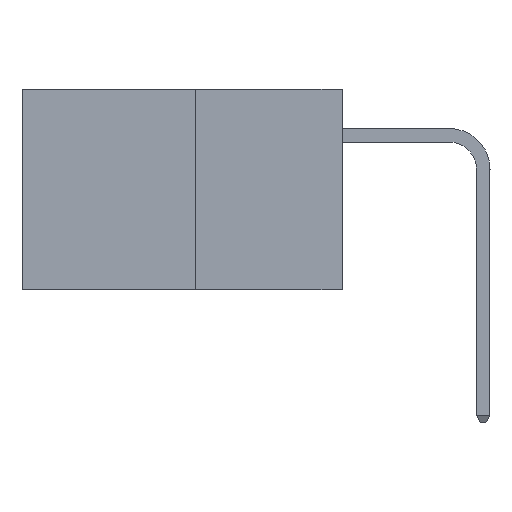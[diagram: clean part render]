
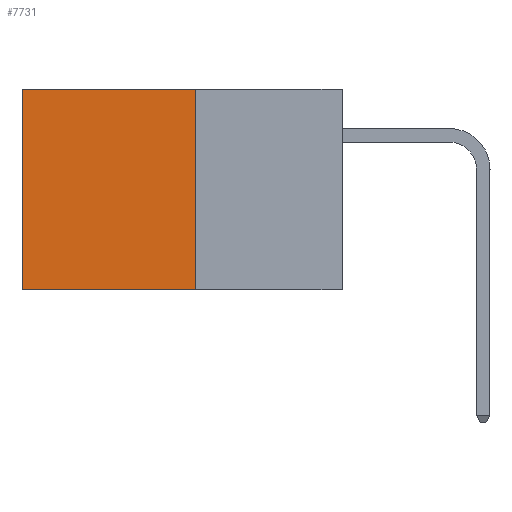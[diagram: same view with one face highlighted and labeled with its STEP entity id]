
A CAD part, left-side view. The second image highlights one B-rep face of the part: STEP entity #7731.
In plain terms, the highlighted planar face has unit normal (-1, 0, 0).
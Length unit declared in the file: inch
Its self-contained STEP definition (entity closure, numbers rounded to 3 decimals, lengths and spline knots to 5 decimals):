
#697 = VECTOR ( 'NONE', #19957, 39.37008 ) ;
#982 = EDGE_LOOP ( 'NONE', ( #28139, #23378, #9929, #31841 ) ) ;
#1897 = VERTEX_POINT ( 'NONE', #28384 ) ;
#2350 = AXIS2_PLACEMENT_3D ( 'NONE', #2389, #30885, #15516 ) ;
#2389 = CARTESIAN_POINT ( 'NONE',  ( 0.277, 0.27, -0.37 ) ) ;
#2440 = LINE ( 'NONE', #23786, #28368 ) ;
#3735 = CARTESIAN_POINT ( 'NONE',  ( 0.277, 0.27, 0. ) ) ;
#6374 = DIRECTION ( 'NONE',  ( 0., 1., 0. ) ) ;
#7622 = PLANE ( 'NONE',  #2350 ) ;
#7630 = LINE ( 'NONE', #22423, #697 ) ;
#7731 = ADVANCED_FACE ( 'NONE', ( #25335 ), #7622, .F. ) ;
#8043 = LINE ( 'NONE', #31973, #27870 ) ;
#9929 = ORIENTED_EDGE ( 'NONE', *, *, #12433, .F. ) ;
#11306 = EDGE_CURVE ( 'NONE', #12851, #21415, #2440, .T. ) ;
#12433 = EDGE_CURVE ( 'NONE', #32656, #12851, #8043, .T. ) ;
#12610 = EDGE_CURVE ( 'NONE', #1897, #21415, #7630, .T. ) ;
#12851 = VERTEX_POINT ( 'NONE', #15685 ) ;
#15516 = DIRECTION ( 'NONE',  ( 0., 0., -1. ) ) ;
#15685 = CARTESIAN_POINT ( 'NONE',  ( 0.277, 0.27, -0.37 ) ) ;
#16673 = CARTESIAN_POINT ( 'NONE',  ( 0.277, 0.27, 0. ) ) ;
#19957 = DIRECTION ( 'NONE',  ( 0., 0., -1. ) ) ;
#21415 = VERTEX_POINT ( 'NONE', #26023 ) ;
#21761 = DIRECTION ( 'NONE',  ( 0., 0., -1. ) ) ;
#22423 = CARTESIAN_POINT ( 'NONE',  ( 0.277, 0.59, -0.37 ) ) ;
#23378 = ORIENTED_EDGE ( 'NONE', *, *, #11306, .F. ) ;
#23786 = CARTESIAN_POINT ( 'NONE',  ( 0.277, 0.27, -0.37 ) ) ;
#25335 = FACE_OUTER_BOUND ( 'NONE', #982, .T. ) ;
#26023 = CARTESIAN_POINT ( 'NONE',  ( 0.277, 0.59, -0.37 ) ) ;
#26364 = DIRECTION ( 'NONE',  ( 0., 1., 0. ) ) ;
#27774 = EDGE_CURVE ( 'NONE', #32656, #1897, #30176, .T. ) ;
#27870 = VECTOR ( 'NONE', #21761, 39.37008 ) ;
#28139 = ORIENTED_EDGE ( 'NONE', *, *, #12610, .T. ) ;
#28368 = VECTOR ( 'NONE', #26364, 39.37008 ) ;
#28384 = CARTESIAN_POINT ( 'NONE',  ( 0.277, 0.59, 0. ) ) ;
#29371 = VECTOR ( 'NONE', #6374, 39.37008 ) ;
#30176 = LINE ( 'NONE', #3735, #29371 ) ;
#30885 = DIRECTION ( 'NONE',  ( 1., 0., 0. ) ) ;
#31841 = ORIENTED_EDGE ( 'NONE', *, *, #27774, .T. ) ;
#31973 = CARTESIAN_POINT ( 'NONE',  ( 0.277, 0.27, -0.37 ) ) ;
#32656 = VERTEX_POINT ( 'NONE', #16673 ) ;
